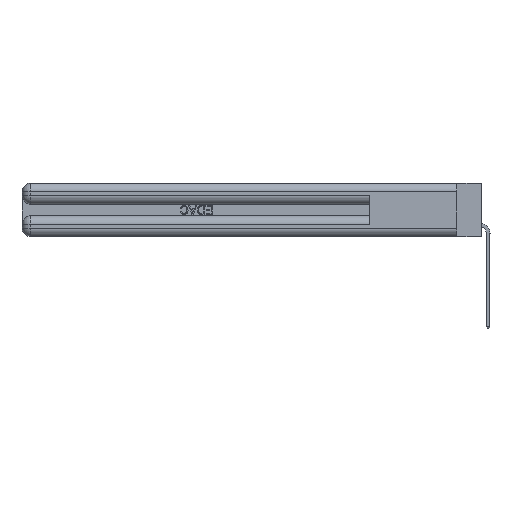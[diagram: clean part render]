
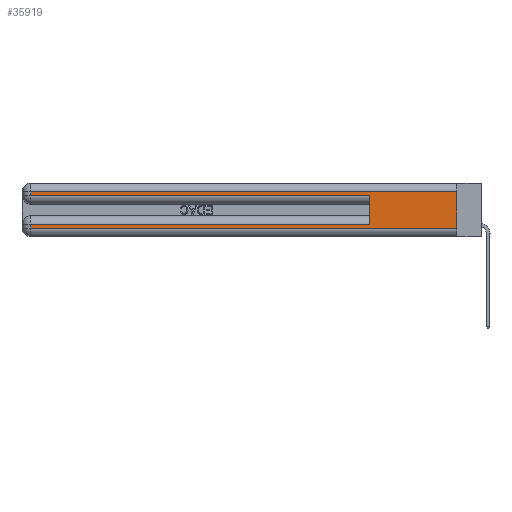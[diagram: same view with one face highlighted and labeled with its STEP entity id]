
A CAD part, left-side view. The second image highlights one B-rep face of the part: STEP entity #35919.
In plain terms, the highlighted planar face has unit normal (-1, 0, 0).
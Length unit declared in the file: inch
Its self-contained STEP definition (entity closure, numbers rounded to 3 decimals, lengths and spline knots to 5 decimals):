
#2 = EDGE_CURVE ( 'NONE', #7331, #3279, #41823, .T. ) ;
#1086 = DIRECTION ( 'NONE',  ( 0., 1., 0. ) ) ;
#2709 = VERTEX_POINT ( 'NONE', #40675 ) ;
#2985 = LINE ( 'NONE', #42301, #33224 ) ;
#3163 = VECTOR ( 'NONE', #38910, 39.37008 ) ;
#3279 = VERTEX_POINT ( 'NONE', #43744 ) ;
#4372 = EDGE_CURVE ( 'NONE', #21899, #6540, #29914, .T. ) ;
#4443 = LINE ( 'NONE', #32499, #16118 ) ;
#5355 = VERTEX_POINT ( 'NONE', #28510 ) ;
#5474 = ORIENTED_EDGE ( 'NONE', *, *, #18366, .T. ) ;
#5689 = ORIENTED_EDGE ( 'NONE', *, *, #22641, .F. ) ;
#5848 = ORIENTED_EDGE ( 'NONE', *, *, #32357, .T. ) ;
#6049 = LINE ( 'NONE', #33624, #42618 ) ;
#6540 = VERTEX_POINT ( 'NONE', #18413 ) ;
#6571 = CARTESIAN_POINT ( 'NONE',  ( 0., 0., 0.285 ) ) ;
#7331 = VERTEX_POINT ( 'NONE', #41606 ) ;
#8965 = CARTESIAN_POINT ( 'NONE',  ( 0., 0., 0.37 ) ) ;
#9438 = VERTEX_POINT ( 'NONE', #36537 ) ;
#11557 = CARTESIAN_POINT ( 'NONE',  ( 0., 0., 0.085 ) ) ;
#11866 = VECTOR ( 'NONE', #33821, 39.37008 ) ;
#12171 = DIRECTION ( 'NONE',  ( 0., -1., 0. ) ) ;
#12622 = CARTESIAN_POINT ( 'NONE',  ( 0., 0., 0.31 ) ) ;
#13221 = EDGE_CURVE ( 'NONE', #3279, #5355, #2985, .T. ) ;
#15647 = EDGE_LOOP ( 'NONE', ( #38090, #27606, #5474, #5848, #5689, #28328, #37754, #22505 ) ) ;
#15963 = AXIS2_PLACEMENT_3D ( 'NONE', #34842, #21172, #38109 ) ;
#16118 = VECTOR ( 'NONE', #25489, 39.37008 ) ;
#17060 = PLANE ( 'NONE',  #15963 ) ;
#18366 = EDGE_CURVE ( 'NONE', #6540, #2709, #4443, .T. ) ;
#18413 = CARTESIAN_POINT ( 'NONE',  ( 0., 2.94, 0.31 ) ) ;
#20139 = VECTOR ( 'NONE', #22150, 39.37008 ) ;
#21172 = DIRECTION ( 'NONE',  ( 1., 0., 0. ) ) ;
#21790 = VERTEX_POINT ( 'NONE', #39891 ) ;
#21899 = VERTEX_POINT ( 'NONE', #27961 ) ;
#22150 = DIRECTION ( 'NONE',  ( 0., -1., 0. ) ) ;
#22505 = ORIENTED_EDGE ( 'NONE', *, *, #41605, .T. ) ;
#22641 = EDGE_CURVE ( 'NONE', #7331, #9438, #6049, .T. ) ;
#23358 = CARTESIAN_POINT ( 'NONE',  ( 0., 0., 0.06 ) ) ;
#23667 = FACE_OUTER_BOUND ( 'NONE', #15647, .T. ) ;
#25489 = DIRECTION ( 'NONE',  ( 0., 0., -1. ) ) ;
#27606 = ORIENTED_EDGE ( 'NONE', *, *, #4372, .T. ) ;
#27961 = CARTESIAN_POINT ( 'NONE',  ( 0., 0., 0.31 ) ) ;
#28006 = LINE ( 'NONE', #8965, #3163 ) ;
#28328 = ORIENTED_EDGE ( 'NONE', *, *, #2, .T. ) ;
#28489 = DIRECTION ( 'NONE',  ( 0., 0., -1. ) ) ;
#28510 = CARTESIAN_POINT ( 'NONE',  ( 0., 2.94, 0.06 ) ) ;
#29914 = LINE ( 'NONE', #12622, #11866 ) ;
#31264 = LINE ( 'NONE', #23358, #20139 ) ;
#31838 = VECTOR ( 'NONE', #12171, 39.37008 ) ;
#32357 = EDGE_CURVE ( 'NONE', #2709, #9438, #41928, .T. ) ;
#32499 = CARTESIAN_POINT ( 'NONE',  ( 0., 2.94, 0.37 ) ) ;
#33224 = VECTOR ( 'NONE', #28489, 39.37008 ) ;
#33624 = CARTESIAN_POINT ( 'NONE',  ( 0., 0.6, 0.145 ) ) ;
#33698 = EDGE_CURVE ( 'NONE', #21899, #21790, #28006, .T. ) ;
#33821 = DIRECTION ( 'NONE',  ( 0., 1., 0. ) ) ;
#34842 = CARTESIAN_POINT ( 'NONE',  ( 0., 0., 0.37 ) ) ;
#34932 = VECTOR ( 'NONE', #1086, 39.37008 ) ;
#35919 = ADVANCED_FACE ( 'NONE', ( #23667 ), #17060, .F. ) ;
#36537 = CARTESIAN_POINT ( 'NONE',  ( 0., 0.6, 0.285 ) ) ;
#37754 = ORIENTED_EDGE ( 'NONE', *, *, #13221, .T. ) ;
#38090 = ORIENTED_EDGE ( 'NONE', *, *, #33698, .F. ) ;
#38109 = DIRECTION ( 'NONE',  ( 0., 0., -1. ) ) ;
#38910 = DIRECTION ( 'NONE',  ( 0., 0., -1. ) ) ;
#39891 = CARTESIAN_POINT ( 'NONE',  ( 0., 0., 0.06 ) ) ;
#40675 = CARTESIAN_POINT ( 'NONE',  ( 0., 2.94, 0.285 ) ) ;
#41605 = EDGE_CURVE ( 'NONE', #5355, #21790, #31264, .T. ) ;
#41606 = CARTESIAN_POINT ( 'NONE',  ( 0., 0.6, 0.085 ) ) ;
#41823 = LINE ( 'NONE', #11557, #34932 ) ;
#41928 = LINE ( 'NONE', #6571, #31838 ) ;
#42301 = CARTESIAN_POINT ( 'NONE',  ( 0., 2.94, 0.37 ) ) ;
#42618 = VECTOR ( 'NONE', #43796, 39.37008 ) ;
#43744 = CARTESIAN_POINT ( 'NONE',  ( 0., 2.94, 0.085 ) ) ;
#43796 = DIRECTION ( 'NONE',  ( 0., 0., 1. ) ) ;
